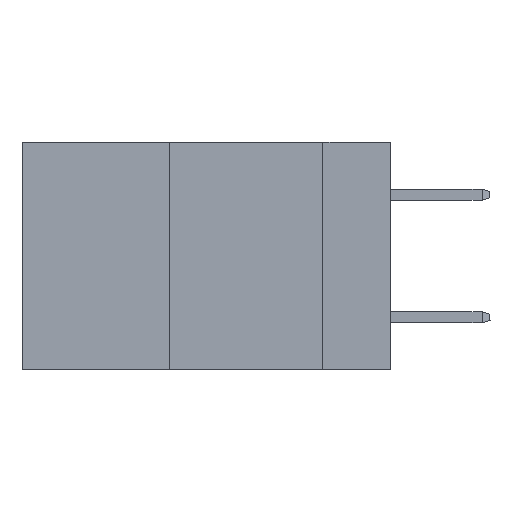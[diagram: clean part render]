
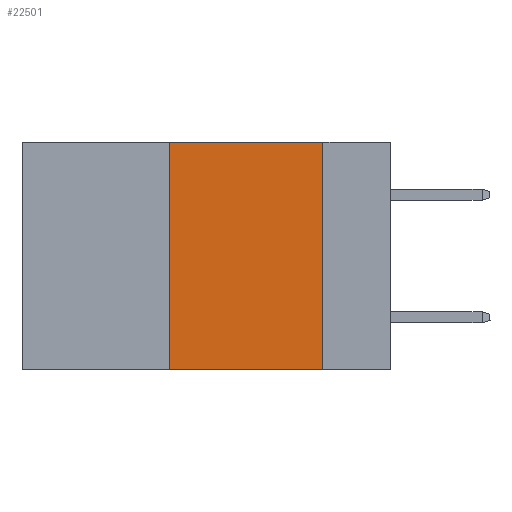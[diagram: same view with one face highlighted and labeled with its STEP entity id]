
A CAD part, left-side view. The second image highlights one B-rep face of the part: STEP entity #22501.
In plain terms, the highlighted planar face has unit normal (-1, 0, 0).
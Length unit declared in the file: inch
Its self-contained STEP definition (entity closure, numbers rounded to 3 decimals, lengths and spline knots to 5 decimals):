
#1133 = CARTESIAN_POINT ( 'NONE',  ( 0., 0.36, 0. ) ) ;
#1274 = CARTESIAN_POINT ( 'NONE',  ( 0., 0.11, -0.37 ) ) ;
#1859 = LINE ( 'NONE', #14953, #19894 ) ;
#2858 = VERTEX_POINT ( 'NONE', #1274 ) ;
#3575 = AXIS2_PLACEMENT_3D ( 'NONE', #16203, #20351, #19993 ) ;
#3748 = CARTESIAN_POINT ( 'NONE',  ( 0., 0.36, -0.37 ) ) ;
#5688 = EDGE_CURVE ( 'NONE', #7245, #24778, #1859, .T. ) ;
#5692 = VECTOR ( 'NONE', #17289, 39.37008 ) ;
#5958 = ORIENTED_EDGE ( 'NONE', *, *, #5688, .F. ) ;
#6273 = DIRECTION ( 'NONE',  ( 0., -1., 0. ) ) ;
#6373 = CARTESIAN_POINT ( 'NONE',  ( 0., 0.11, 0. ) ) ;
#6896 = VECTOR ( 'NONE', #6273, 39.37008 ) ;
#7245 = VERTEX_POINT ( 'NONE', #3748 ) ;
#8350 = CARTESIAN_POINT ( 'NONE',  ( 0., 0.11, 0. ) ) ;
#10196 = LINE ( 'NONE', #13138, #5692 ) ;
#10751 = EDGE_CURVE ( 'NONE', #24778, #14313, #22030, .T. ) ;
#10793 = FACE_OUTER_BOUND ( 'NONE', #17057, .T. ) ;
#10917 = ORIENTED_EDGE ( 'NONE', *, *, #15493, .F. ) ;
#13138 = CARTESIAN_POINT ( 'NONE',  ( 0., 0.6, -0.37 ) ) ;
#13723 = LINE ( 'NONE', #8350, #16626 ) ;
#13944 = ORIENTED_EDGE ( 'NONE', *, *, #15284, .T. ) ;
#14313 = VERTEX_POINT ( 'NONE', #6373 ) ;
#14621 = CARTESIAN_POINT ( 'NONE',  ( 0., 0.6, 0. ) ) ;
#14953 = CARTESIAN_POINT ( 'NONE',  ( 0., 0.36, 0. ) ) ;
#15284 = EDGE_CURVE ( 'NONE', #7245, #2858, #10196, .T. ) ;
#15493 = EDGE_CURVE ( 'NONE', #14313, #2858, #13723, .T. ) ;
#16203 = CARTESIAN_POINT ( 'NONE',  ( 0., 0.6, 0. ) ) ;
#16626 = VECTOR ( 'NONE', #24779, 39.37008 ) ;
#17057 = EDGE_LOOP ( 'NONE', ( #10917, #24788, #5958, #13944 ) ) ;
#17289 = DIRECTION ( 'NONE',  ( 0., -1., 0. ) ) ;
#19894 = VECTOR ( 'NONE', #20828, 39.37008 ) ;
#19993 = DIRECTION ( 'NONE',  ( 0., 0., -1. ) ) ;
#20351 = DIRECTION ( 'NONE',  ( 1., 0., 0. ) ) ;
#20828 = DIRECTION ( 'NONE',  ( 0., 0., 1. ) ) ;
#22030 = LINE ( 'NONE', #14621, #6896 ) ;
#22501 = ADVANCED_FACE ( 'NONE', ( #10793 ), #26238, .F. ) ;
#24778 = VERTEX_POINT ( 'NONE', #1133 ) ;
#24779 = DIRECTION ( 'NONE',  ( 0., 0., -1. ) ) ;
#24788 = ORIENTED_EDGE ( 'NONE', *, *, #10751, .F. ) ;
#26238 = PLANE ( 'NONE',  #3575 ) ;
